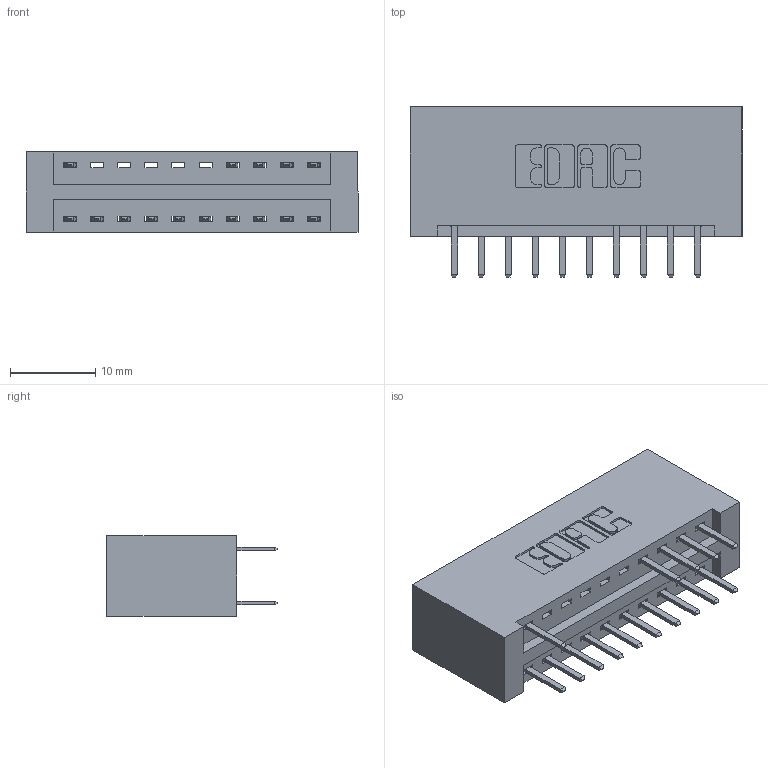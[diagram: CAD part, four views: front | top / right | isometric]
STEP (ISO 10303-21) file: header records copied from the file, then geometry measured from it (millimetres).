
FILE_DESCRIPTION (( 'STEP AP203' ), '1' );
FILE_NAME ('346-020-520-201.STEP', '2018-08-20T10:57:45', ( '' ), ( '' ), 'SwSTEP 2.0', 'SolidWorks 2016', '' );
FILE_SCHEMA (( 'CONFIG_CONTROL_DESIGN' ));
Length unit declared in the file: inch
Products named in the file (3): 346 Part_No Mounting Lugs; 345-292-001_345-293-120; 346-020-520-201
Assembly tree (16 placements, depth 2):
  346-020-520-201
    346 Part_No Mounting Lugs
    345-292-001_345-293-120  x15
Bounding box: 38.99 x 20.02 x 9.4 mm (x, y, z)
Volume: 4075.1 mm3; surface area: 4986.8 mm2
Topology: 16 solids, 16 shells, 984 faces, 2855 edges, 1862 vertices
Faces by surface type: plane 652, cylinder 332
Entity records: 10511 total; most frequent: CARTESIAN_POINT 1807, ORIENTED_EDGE 1734, DIRECTION 1621, EDGE_CURVE 867, VECTOR 699, LINE 699, VERTEX_POINT 574, AXIS2_PLACEMENT_3D 461
